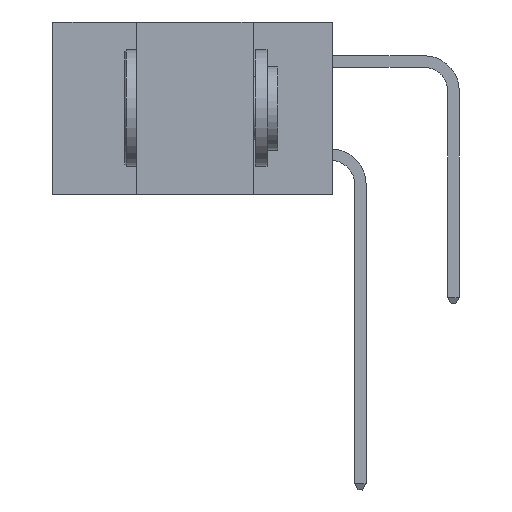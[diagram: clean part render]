
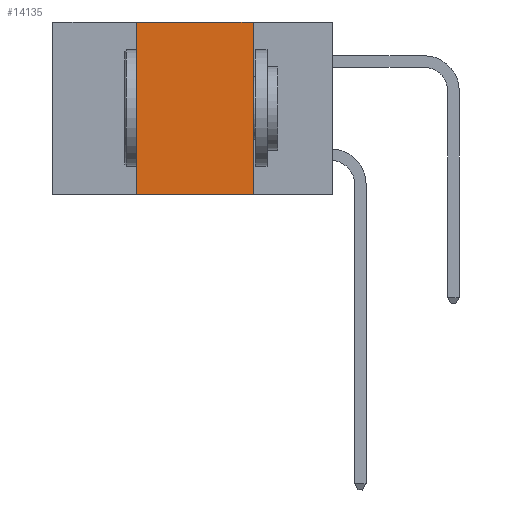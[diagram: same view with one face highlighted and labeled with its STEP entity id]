
A CAD part, left-side view. The second image highlights one B-rep face of the part: STEP entity #14135.
In plain terms, the highlighted planar face has unit normal (-1, 0, 0).
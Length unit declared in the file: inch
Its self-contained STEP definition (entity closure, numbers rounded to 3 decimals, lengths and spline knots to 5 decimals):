
#106 = VERTEX_POINT ( 'NONE', #15501 ) ;
#1009 = ORIENTED_EDGE ( 'NONE', *, *, #28691, .T. ) ;
#1176 = DIRECTION ( 'NONE',  ( 0., 0., -1. ) ) ;
#1363 = LINE ( 'NONE', #28722, #12738 ) ;
#2145 = ORIENTED_EDGE ( 'NONE', *, *, #10448, .F. ) ;
#2336 = DIRECTION ( 'NONE',  ( 0., 0., -1. ) ) ;
#5021 = LINE ( 'NONE', #25762, #11752 ) ;
#5515 = CARTESIAN_POINT ( 'NONE',  ( 0., 0.42, -0.37 ) ) ;
#8342 = DIRECTION ( 'NONE',  ( 0., 0., 1. ) ) ;
#8463 = VECTOR ( 'NONE', #21347, 39.37008 ) ;
#8542 = ORIENTED_EDGE ( 'NONE', *, *, #28064, .F. ) ;
#8791 = VERTEX_POINT ( 'NONE', #5515 ) ;
#10017 = VECTOR ( 'NONE', #2336, 39.37008 ) ;
#10448 = EDGE_CURVE ( 'NONE', #14362, #106, #26544, .T. ) ;
#11372 = CARTESIAN_POINT ( 'NONE',  ( 0., 0.17, 0. ) ) ;
#11433 = LINE ( 'NONE', #11372, #10017 ) ;
#11752 = VECTOR ( 'NONE', #28039, 39.37008 ) ;
#12738 = VECTOR ( 'NONE', #8342, 39.37008 ) ;
#13135 = VERTEX_POINT ( 'NONE', #20384 ) ;
#14135 = ADVANCED_FACE ( 'NONE', ( #16310 ), #28344, .F. ) ;
#14293 = EDGE_CURVE ( 'NONE', #8791, #14362, #1363, .T. ) ;
#14362 = VERTEX_POINT ( 'NONE', #26755 ) ;
#14789 = DIRECTION ( 'NONE',  ( 1., 0., 0. ) ) ;
#15501 = CARTESIAN_POINT ( 'NONE',  ( 0., 0.17, 0. ) ) ;
#16310 = FACE_OUTER_BOUND ( 'NONE', #16687, .T. ) ;
#16687 = EDGE_LOOP ( 'NONE', ( #8542, #2145, #27711, #1009 ) ) ;
#19068 = CARTESIAN_POINT ( 'NONE',  ( 0., 0.6, 0. ) ) ;
#20384 = CARTESIAN_POINT ( 'NONE',  ( 0., 0.17, -0.37 ) ) ;
#21294 = AXIS2_PLACEMENT_3D ( 'NONE', #21527, #14789, #1176 ) ;
#21347 = DIRECTION ( 'NONE',  ( 0., -1., 0. ) ) ;
#21527 = CARTESIAN_POINT ( 'NONE',  ( 0., 0.6, 0. ) ) ;
#25762 = CARTESIAN_POINT ( 'NONE',  ( 0., 0.6, -0.37 ) ) ;
#26544 = LINE ( 'NONE', #19068, #8463 ) ;
#26755 = CARTESIAN_POINT ( 'NONE',  ( 0., 0.42, 0. ) ) ;
#27711 = ORIENTED_EDGE ( 'NONE', *, *, #14293, .F. ) ;
#28039 = DIRECTION ( 'NONE',  ( 0., -1., 0. ) ) ;
#28064 = EDGE_CURVE ( 'NONE', #106, #13135, #11433, .T. ) ;
#28344 = PLANE ( 'NONE',  #21294 ) ;
#28691 = EDGE_CURVE ( 'NONE', #8791, #13135, #5021, .T. ) ;
#28722 = CARTESIAN_POINT ( 'NONE',  ( 0., 0.42, 0. ) ) ;
